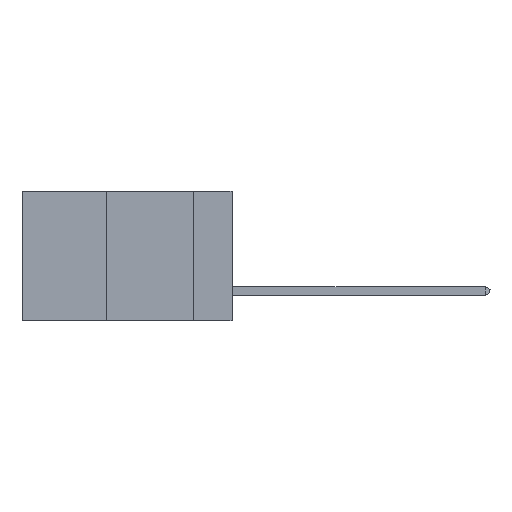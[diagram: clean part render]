
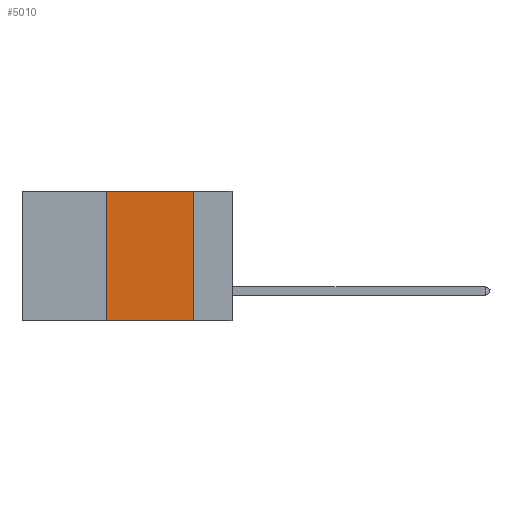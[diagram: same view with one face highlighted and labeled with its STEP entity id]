
A CAD part, left-side view. The second image highlights one B-rep face of the part: STEP entity #5010.
In plain terms, the highlighted planar face has unit normal (-1, 0, 0).
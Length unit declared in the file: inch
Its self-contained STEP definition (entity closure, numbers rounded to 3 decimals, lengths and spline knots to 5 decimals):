
#172 = EDGE_LOOP ( 'NONE', ( #27057, #26586, #9047, #22838 ) ) ;
#224 = AXIS2_PLACEMENT_3D ( 'NONE', #29752, #9797, #14761 ) ;
#3570 = VECTOR ( 'NONE', #13657, 39.37008 ) ;
#5010 = ADVANCED_FACE ( 'NONE', ( #5989 ), #24905, .F. ) ;
#5367 = LINE ( 'NONE', #12177, #7304 ) ;
#5989 = FACE_OUTER_BOUND ( 'NONE', #172, .T. ) ;
#6340 = VERTEX_POINT ( 'NONE', #7884 ) ;
#6475 = CARTESIAN_POINT ( 'NONE',  ( 0., 0.11, 0. ) ) ;
#6693 = CARTESIAN_POINT ( 'NONE',  ( 0., 0.36, 0. ) ) ;
#7304 = VECTOR ( 'NONE', #17077, 39.37008 ) ;
#7562 = LINE ( 'NONE', #23157, #28537 ) ;
#7884 = CARTESIAN_POINT ( 'NONE',  ( 0., 0.36, -0.37 ) ) ;
#8001 = DIRECTION ( 'NONE',  ( 0., 0., -1. ) ) ;
#8416 = CARTESIAN_POINT ( 'NONE',  ( 0., 0.11, -0.37 ) ) ;
#9047 = ORIENTED_EDGE ( 'NONE', *, *, #14859, .F. ) ;
#9797 = DIRECTION ( 'NONE',  ( 1., 0., 0. ) ) ;
#10575 = EDGE_CURVE ( 'NONE', #6340, #24064, #7562, .T. ) ;
#11298 = LINE ( 'NONE', #22825, #30304 ) ;
#11717 = LINE ( 'NONE', #18514, #3570 ) ;
#12177 = CARTESIAN_POINT ( 'NONE',  ( 0., 0.36, 0. ) ) ;
#12347 = VERTEX_POINT ( 'NONE', #6475 ) ;
#13052 = EDGE_CURVE ( 'NONE', #12347, #24064, #11298, .T. ) ;
#13657 = DIRECTION ( 'NONE',  ( 0., -1., 0. ) ) ;
#14057 = DIRECTION ( 'NONE',  ( 0., -1., 0. ) ) ;
#14761 = DIRECTION ( 'NONE',  ( 0., 0., -1. ) ) ;
#14859 = EDGE_CURVE ( 'NONE', #6340, #16493, #5367, .T. ) ;
#16493 = VERTEX_POINT ( 'NONE', #6693 ) ;
#17077 = DIRECTION ( 'NONE',  ( 0., 0., 1. ) ) ;
#18514 = CARTESIAN_POINT ( 'NONE',  ( 0., 0.6, 0. ) ) ;
#19359 = EDGE_CURVE ( 'NONE', #16493, #12347, #11717, .T. ) ;
#22825 = CARTESIAN_POINT ( 'NONE',  ( 0., 0.11, 0. ) ) ;
#22838 = ORIENTED_EDGE ( 'NONE', *, *, #10575, .T. ) ;
#23157 = CARTESIAN_POINT ( 'NONE',  ( 0., 0.6, -0.37 ) ) ;
#24064 = VERTEX_POINT ( 'NONE', #8416 ) ;
#24905 = PLANE ( 'NONE',  #224 ) ;
#26586 = ORIENTED_EDGE ( 'NONE', *, *, #19359, .F. ) ;
#27057 = ORIENTED_EDGE ( 'NONE', *, *, #13052, .F. ) ;
#28537 = VECTOR ( 'NONE', #14057, 39.37008 ) ;
#29752 = CARTESIAN_POINT ( 'NONE',  ( 0., 0.6, 0. ) ) ;
#30304 = VECTOR ( 'NONE', #8001, 39.37008 ) ;
